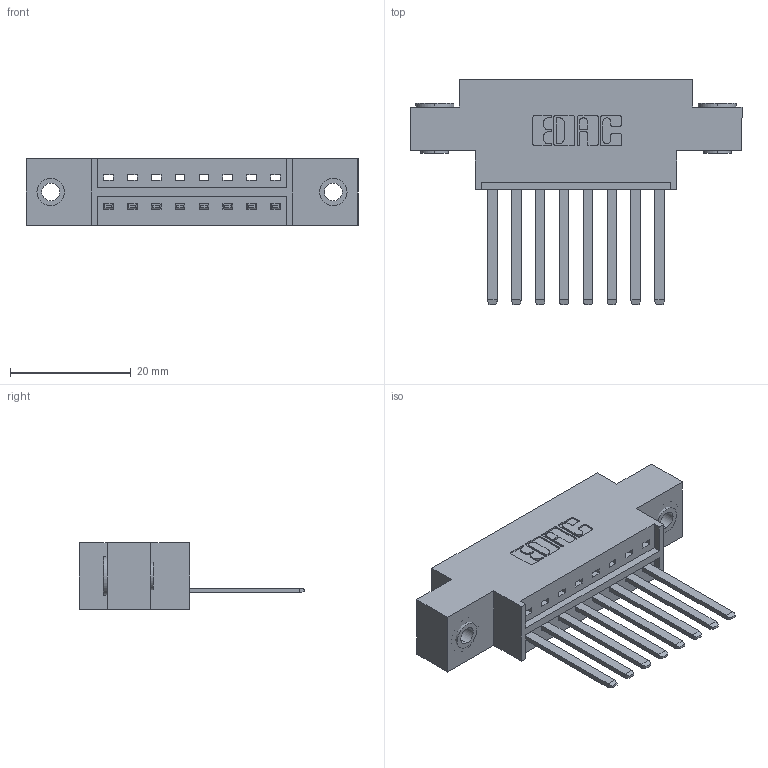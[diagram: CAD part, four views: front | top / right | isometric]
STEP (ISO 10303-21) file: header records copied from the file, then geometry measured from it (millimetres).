
FILE_DESCRIPTION (( 'STEP AP203' ), '1' );
FILE_NAME ('336-008-541-603.STEP', '2020-08-07T19:20:55', ( '' ), ( '' ), 'SwSTEP 2.0', 'SolidWorks 2020', '' );
FILE_SCHEMA (( 'CONFIG_CONTROL_DESIGN' ));
Length unit declared in the file: inch
Products named in the file (4): 336 Part_Offset - .156 Dia - TH; 336-290-001_336-290-541; 336-008-541-603; 345-250-002_345-250-002-102
Assembly tree (11 placements, depth 2):
  336-008-541-603
    336 Part_Offset - .156 Dia - TH
    336-290-001_336-290-541  x8
    345-250-002_345-250-002-102  x2
Bounding box: 55.09 x 37.34 x 11.1 mm (x, y, z)
Volume: 7063.4 mm3; surface area: 7565.4 mm2
Topology: 11 solids, 11 shells, 556 faces, 1631 edges, 1078 vertices
Faces by surface type: plane 356, cylinder 192, cone 8
Entity records: 10845 total; most frequent: CARTESIAN_POINT 1948, ORIENTED_EDGE 1786, DIRECTION 1647, EDGE_CURVE 893, VECTOR 737, LINE 737, VERTEX_POINT 592, AXIS2_PLACEMENT_3D 455
